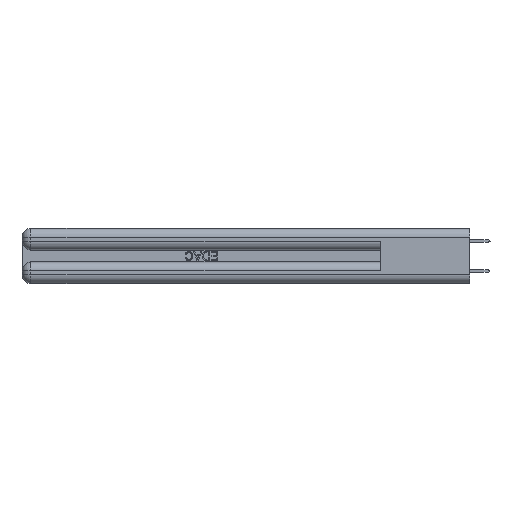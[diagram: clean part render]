
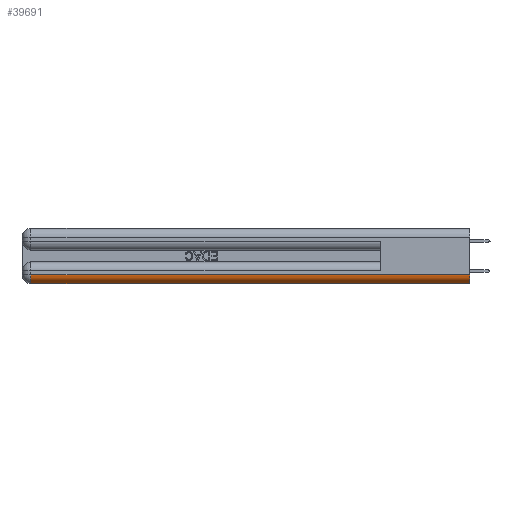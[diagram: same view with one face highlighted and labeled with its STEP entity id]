
A CAD part, left-side view. The second image highlights one B-rep face of the part: STEP entity #39691.
In plain terms, the highlighted cylindrical face has radius 1.524 mm (diameter 3.048 mm), a partial arc.
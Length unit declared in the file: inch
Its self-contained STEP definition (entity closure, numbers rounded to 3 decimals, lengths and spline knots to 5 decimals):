
#666 = ORIENTED_EDGE ( 'NONE', *, *, #24204, .F. ) ;
#696 = CYLINDRICAL_SURFACE ( 'NONE', #3976, 0.06 ) ;
#3956 = CARTESIAN_POINT ( 'NONE',  ( 0.06, 3., 0. ) ) ;
#3976 = AXIS2_PLACEMENT_3D ( 'NONE', #34345, #40518, #24405 ) ;
#5778 = ORIENTED_EDGE ( 'NONE', *, *, #30750, .F. ) ;
#11962 = CARTESIAN_POINT ( 'NONE',  ( 0.06, 2.94, 0. ) ) ;
#13167 = VERTEX_POINT ( 'NONE', #39559 ) ;
#15714 = ORIENTED_EDGE ( 'NONE', *, *, #40749, .F. ) ;
#18748 = VECTOR ( 'NONE', #42367, 39.37008 ) ;
#20266 = CARTESIAN_POINT ( 'NONE',  ( 0.06, 2.94, 0.06 ) ) ;
#21288 = CIRCLE ( 'NONE', #24776, 0.06 ) ;
#22858 = CARTESIAN_POINT ( 'NONE',  ( 0.06, 0., 0.06 ) ) ;
#23068 = DIRECTION ( 'NONE',  ( 0., -1., 0. ) ) ;
#23567 = DIRECTION ( 'NONE',  ( 0., 1., 0. ) ) ;
#23705 = VERTEX_POINT ( 'NONE', #11962 ) ;
#24204 = EDGE_CURVE ( 'NONE', #23705, #41680, #25921, .T. ) ;
#24405 = DIRECTION ( 'NONE',  ( 0., 0., 1. ) ) ;
#24776 = AXIS2_PLACEMENT_3D ( 'NONE', #22858, #23068, #30332 ) ;
#25921 = CIRCLE ( 'NONE', #26610, 0.06 ) ;
#26465 = DIRECTION ( 'NONE',  ( 0., 0., 1. ) ) ;
#26610 = AXIS2_PLACEMENT_3D ( 'NONE', #20266, #23567, #26465 ) ;
#30332 = DIRECTION ( 'NONE',  ( 0., 0., 1. ) ) ;
#30750 = EDGE_CURVE ( 'NONE', #41712, #13167, #21288, .T. ) ;
#30876 = EDGE_CURVE ( 'NONE', #13167, #23705, #31613, .T. ) ;
#31134 = VECTOR ( 'NONE', #34083, 39.37008 ) ;
#31613 = LINE ( 'NONE', #3956, #31134 ) ;
#32042 = ORIENTED_EDGE ( 'NONE', *, *, #30876, .F. ) ;
#34083 = DIRECTION ( 'NONE',  ( 0., 1., 0. ) ) ;
#34243 = CARTESIAN_POINT ( 'NONE',  ( 0., 0., 0.06 ) ) ;
#34345 = CARTESIAN_POINT ( 'NONE',  ( 0.06, 0., 0.06 ) ) ;
#37630 = FACE_OUTER_BOUND ( 'NONE', #42825, .T. ) ;
#39559 = CARTESIAN_POINT ( 'NONE',  ( 0.06, 0., 0. ) ) ;
#39691 = ADVANCED_FACE ( 'NONE', ( #37630 ), #696, .T. ) ;
#40518 = DIRECTION ( 'NONE',  ( 0., 1., 0. ) ) ;
#40749 = EDGE_CURVE ( 'NONE', #41680, #41712, #41715, .T. ) ;
#41514 = CARTESIAN_POINT ( 'NONE',  ( 0., 2.94, 0.06 ) ) ;
#41680 = VERTEX_POINT ( 'NONE', #41514 ) ;
#41712 = VERTEX_POINT ( 'NONE', #34243 ) ;
#41715 = LINE ( 'NONE', #41933, #18748 ) ;
#41933 = CARTESIAN_POINT ( 'NONE',  ( 0., 0., 0.06 ) ) ;
#42367 = DIRECTION ( 'NONE',  ( 0., -1., 0. ) ) ;
#42825 = EDGE_LOOP ( 'NONE', ( #5778, #15714, #666, #32042 ) ) ;
